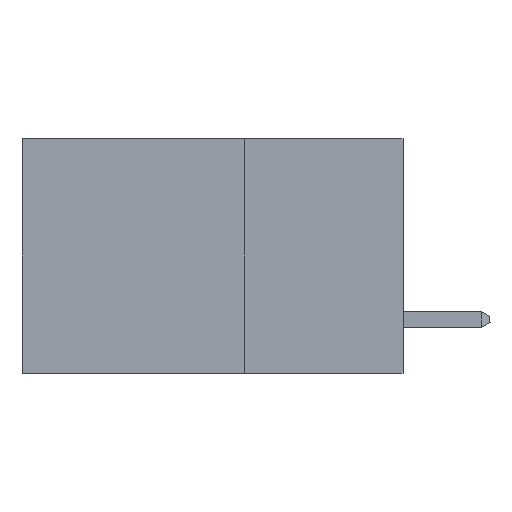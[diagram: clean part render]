
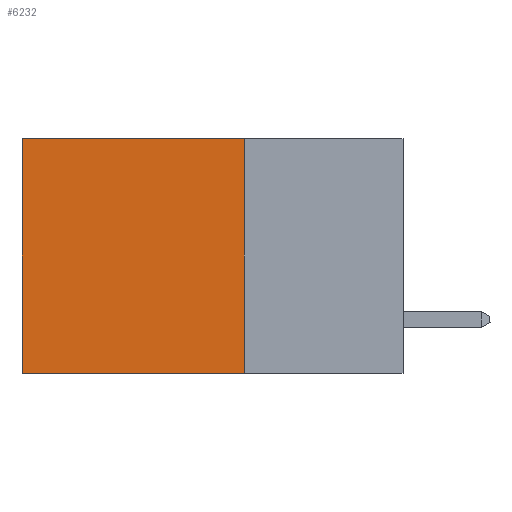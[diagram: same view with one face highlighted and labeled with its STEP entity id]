
A CAD part, left-side view. The second image highlights one B-rep face of the part: STEP entity #6232.
In plain terms, the highlighted planar face has unit normal (-1, 0, 0).
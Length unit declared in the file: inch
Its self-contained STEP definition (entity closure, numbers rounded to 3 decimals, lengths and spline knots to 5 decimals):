
#16 = EDGE_CURVE ( 'NONE', #2248, #10551, #3147, .T. ) ;
#226 = DIRECTION ( 'NONE',  ( 0., 1., 0. ) ) ;
#487 = VERTEX_POINT ( 'NONE', #1571 ) ;
#710 = EDGE_CURVE ( 'NONE', #2248, #2897, #8301, .T. ) ;
#939 = EDGE_CURVE ( 'NONE', #10551, #487, #2315, .T. ) ;
#1313 = PLANE ( 'NONE',  #8315 ) ;
#1565 = ORIENTED_EDGE ( 'NONE', *, *, #16, .F. ) ;
#1571 = CARTESIAN_POINT ( 'NONE',  ( 0.2875, 0.6, -0.37 ) ) ;
#1696 = CARTESIAN_POINT ( 'NONE',  ( 0.2875, 0.25, -0.37 ) ) ;
#1789 = CARTESIAN_POINT ( 'NONE',  ( 0.2875, 0.6, 0. ) ) ;
#2248 = VERTEX_POINT ( 'NONE', #8501 ) ;
#2315 = LINE ( 'NONE', #5535, #2853 ) ;
#2516 = ORIENTED_EDGE ( 'NONE', *, *, #939, .F. ) ;
#2652 = VECTOR ( 'NONE', #10016, 39.37008 ) ;
#2853 = VECTOR ( 'NONE', #226, 39.37008 ) ;
#2897 = VERTEX_POINT ( 'NONE', #1789 ) ;
#3071 = CARTESIAN_POINT ( 'NONE',  ( 0.2875, 0.6, 0. ) ) ;
#3147 = LINE ( 'NONE', #7906, #7095 ) ;
#4488 = DIRECTION ( 'NONE',  ( 0., 1., 0. ) ) ;
#4782 = EDGE_CURVE ( 'NONE', #2897, #487, #9437, .T. ) ;
#5535 = CARTESIAN_POINT ( 'NONE',  ( 0.2875, 0.25, -0.37 ) ) ;
#5726 = DIRECTION ( 'NONE',  ( 0., 0., -1. ) ) ;
#6001 = VECTOR ( 'NONE', #4488, 39.37008 ) ;
#6231 = ORIENTED_EDGE ( 'NONE', *, *, #710, .T. ) ;
#6232 = ADVANCED_FACE ( 'NONE', ( #6236 ), #1313, .F. ) ;
#6236 = FACE_OUTER_BOUND ( 'NONE', #10688, .T. ) ;
#6970 = DIRECTION ( 'NONE',  ( 0., 0., -1. ) ) ;
#7095 = VECTOR ( 'NONE', #6970, 39.37008 ) ;
#7446 = DIRECTION ( 'NONE',  ( 1., 0., 0. ) ) ;
#7906 = CARTESIAN_POINT ( 'NONE',  ( 0.2875, 0.25, 0. ) ) ;
#7986 = CARTESIAN_POINT ( 'NONE',  ( 0.2875, 0.25, 0. ) ) ;
#8301 = LINE ( 'NONE', #7986, #6001 ) ;
#8315 = AXIS2_PLACEMENT_3D ( 'NONE', #10036, #7446, #5726 ) ;
#8501 = CARTESIAN_POINT ( 'NONE',  ( 0.2875, 0.25, 0. ) ) ;
#8608 = ORIENTED_EDGE ( 'NONE', *, *, #4782, .T. ) ;
#9437 = LINE ( 'NONE', #3071, #2652 ) ;
#10016 = DIRECTION ( 'NONE',  ( 0., 0., -1. ) ) ;
#10036 = CARTESIAN_POINT ( 'NONE',  ( 0.2875, 0.25, 0. ) ) ;
#10551 = VERTEX_POINT ( 'NONE', #1696 ) ;
#10688 = EDGE_LOOP ( 'NONE', ( #8608, #2516, #1565, #6231 ) ) ;
